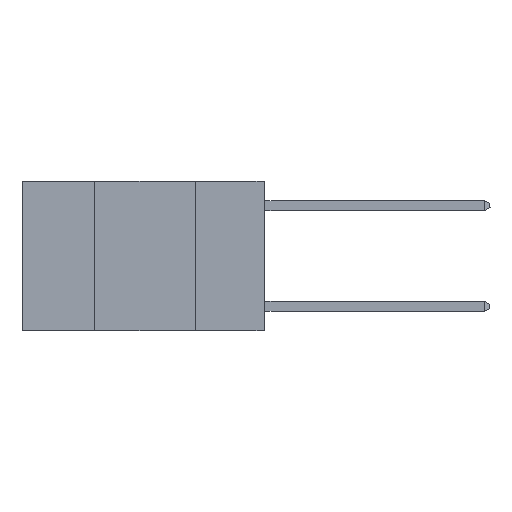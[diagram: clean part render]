
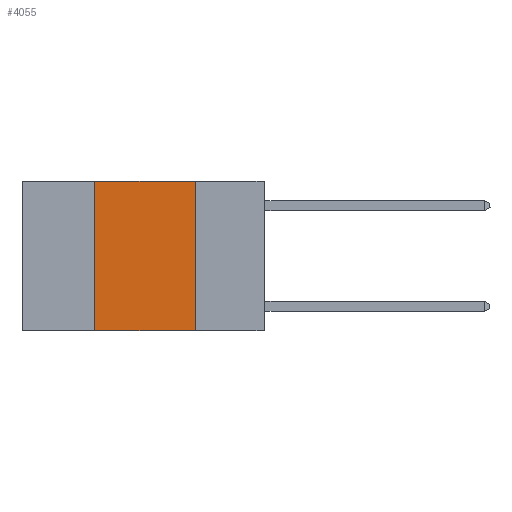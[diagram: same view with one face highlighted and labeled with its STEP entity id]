
A CAD part, left-side view. The second image highlights one B-rep face of the part: STEP entity #4055.
In plain terms, the highlighted planar face has unit normal (-1, 0, 0).
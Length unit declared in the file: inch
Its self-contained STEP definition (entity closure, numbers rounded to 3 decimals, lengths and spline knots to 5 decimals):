
#308 = CARTESIAN_POINT ( 'NONE',  ( 0., 0.17, -0.37 ) ) ;
#387 = CARTESIAN_POINT ( 'NONE',  ( 0., 0.17, 0. ) ) ;
#886 = CARTESIAN_POINT ( 'NONE',  ( 0., 0.42, 0. ) ) ;
#914 = CARTESIAN_POINT ( 'NONE',  ( 0., 0.42, -0.37 ) ) ;
#1042 = VECTOR ( 'NONE', #2138, 39.37008 ) ;
#1336 = ORIENTED_EDGE ( 'NONE', *, *, #4945, .F. ) ;
#1356 = CARTESIAN_POINT ( 'NONE',  ( 0., 0.6, -0.37 ) ) ;
#1388 = VECTOR ( 'NONE', #6192, 39.37008 ) ;
#1414 = LINE ( 'NONE', #7924, #5917 ) ;
#1756 = EDGE_LOOP ( 'NONE', ( #1336, #3282, #6091, #10232 ) ) ;
#2138 = DIRECTION ( 'NONE',  ( 0., -1., 0. ) ) ;
#2786 = EDGE_CURVE ( 'NONE', #9877, #10139, #9179, .T. ) ;
#2907 = DIRECTION ( 'NONE',  ( 0., 0., 1. ) ) ;
#2932 = VERTEX_POINT ( 'NONE', #914 ) ;
#3064 = PLANE ( 'NONE',  #4701 ) ;
#3282 = ORIENTED_EDGE ( 'NONE', *, *, #2786, .F. ) ;
#3984 = EDGE_CURVE ( 'NONE', #2932, #9877, #1414, .T. ) ;
#4055 = ADVANCED_FACE ( 'NONE', ( #9138 ), #3064, .F. ) ;
#4701 = AXIS2_PLACEMENT_3D ( 'NONE', #7250, #9595, #4782 ) ;
#4782 = DIRECTION ( 'NONE',  ( 0., 0., -1. ) ) ;
#4945 = EDGE_CURVE ( 'NONE', #10139, #6612, #5309, .T. ) ;
#5309 = LINE ( 'NONE', #387, #1388 ) ;
#5917 = VECTOR ( 'NONE', #2907, 39.37008 ) ;
#6091 = ORIENTED_EDGE ( 'NONE', *, *, #3984, .F. ) ;
#6192 = DIRECTION ( 'NONE',  ( 0., 0., -1. ) ) ;
#6612 = VERTEX_POINT ( 'NONE', #308 ) ;
#6824 = VECTOR ( 'NONE', #7958, 39.37008 ) ;
#6905 = CARTESIAN_POINT ( 'NONE',  ( 0., 0.17, 0. ) ) ;
#6934 = EDGE_CURVE ( 'NONE', #2932, #6612, #9706, .T. ) ;
#7146 = CARTESIAN_POINT ( 'NONE',  ( 0., 0.6, 0. ) ) ;
#7250 = CARTESIAN_POINT ( 'NONE',  ( 0., 0.6, 0. ) ) ;
#7924 = CARTESIAN_POINT ( 'NONE',  ( 0., 0.42, 0. ) ) ;
#7958 = DIRECTION ( 'NONE',  ( 0., -1., 0. ) ) ;
#9138 = FACE_OUTER_BOUND ( 'NONE', #1756, .T. ) ;
#9179 = LINE ( 'NONE', #7146, #6824 ) ;
#9595 = DIRECTION ( 'NONE',  ( 1., 0., 0. ) ) ;
#9706 = LINE ( 'NONE', #1356, #1042 ) ;
#9877 = VERTEX_POINT ( 'NONE', #886 ) ;
#10139 = VERTEX_POINT ( 'NONE', #6905 ) ;
#10232 = ORIENTED_EDGE ( 'NONE', *, *, #6934, .T. ) ;
